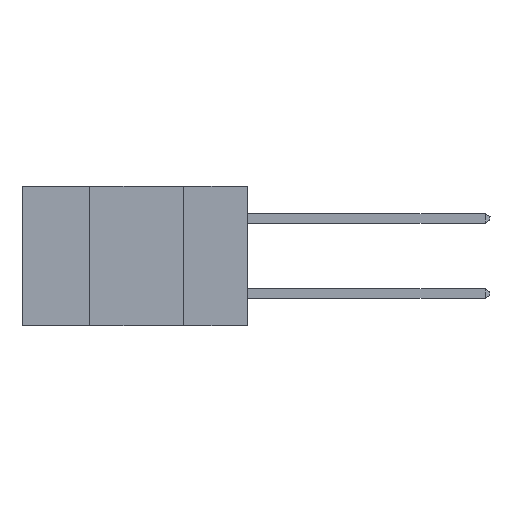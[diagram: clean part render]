
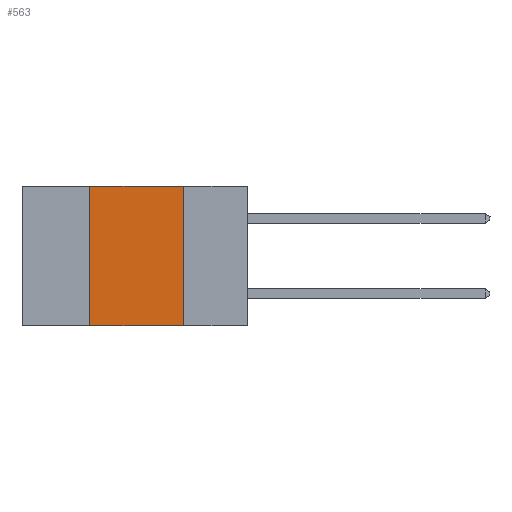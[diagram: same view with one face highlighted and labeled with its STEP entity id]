
A CAD part, left-side view. The second image highlights one B-rep face of the part: STEP entity #563.
In plain terms, the highlighted planar face has unit normal (-1, 0, 0).
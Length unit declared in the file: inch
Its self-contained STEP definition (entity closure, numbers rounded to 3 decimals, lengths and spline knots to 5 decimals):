
#563 = ADVANCED_FACE ( 'NONE', ( #631 ), #5371, .F. ) ;
#631 = FACE_OUTER_BOUND ( 'NONE', #15183, .T. ) ;
#861 = LINE ( 'NONE', #5600, #4841 ) ;
#929 = CARTESIAN_POINT ( 'NONE',  ( 0., 0.17, -0.37 ) ) ;
#1755 = ORIENTED_EDGE ( 'NONE', *, *, #13039, .F. ) ;
#1930 = LINE ( 'NONE', #14336, #5604 ) ;
#2170 = VERTEX_POINT ( 'NONE', #2237 ) ;
#2237 = CARTESIAN_POINT ( 'NONE',  ( 0., 0.42, -0.37 ) ) ;
#2641 = AXIS2_PLACEMENT_3D ( 'NONE', #10121, #14870, #3263 ) ;
#3263 = DIRECTION ( 'NONE',  ( 0., 0., -1. ) ) ;
#3550 = ORIENTED_EDGE ( 'NONE', *, *, #6660, .T. ) ;
#3672 = DIRECTION ( 'NONE',  ( 0., -1., 0. ) ) ;
#4181 = CARTESIAN_POINT ( 'NONE',  ( 0., 0.17, 0. ) ) ;
#4212 = LINE ( 'NONE', #929, #6232 ) ;
#4841 = VECTOR ( 'NONE', #6774, 39.37008 ) ;
#5371 = PLANE ( 'NONE',  #2641 ) ;
#5600 = CARTESIAN_POINT ( 'NONE',  ( 0., 0.42, -0.37 ) ) ;
#5604 = VECTOR ( 'NONE', #3672, 39.37008 ) ;
#6186 = CARTESIAN_POINT ( 'NONE',  ( 0., 0.6, 0. ) ) ;
#6232 = VECTOR ( 'NONE', #14010, 39.37008 ) ;
#6468 = ORIENTED_EDGE ( 'NONE', *, *, #8376, .F. ) ;
#6473 = VERTEX_POINT ( 'NONE', #4181 ) ;
#6573 = CARTESIAN_POINT ( 'NONE',  ( 0., 0.17, -0.37 ) ) ;
#6660 = EDGE_CURVE ( 'NONE', #2170, #8579, #1930, .T. ) ;
#6774 = DIRECTION ( 'NONE',  ( 0., 0., 1. ) ) ;
#8376 = EDGE_CURVE ( 'NONE', #15079, #6473, #13581, .T. ) ;
#8579 = VERTEX_POINT ( 'NONE', #6573 ) ;
#9232 = ORIENTED_EDGE ( 'NONE', *, *, #9540, .F. ) ;
#9540 = EDGE_CURVE ( 'NONE', #6473, #8579, #4212, .T. ) ;
#10121 = CARTESIAN_POINT ( 'NONE',  ( 0., 0.6, 0. ) ) ;
#11269 = VECTOR ( 'NONE', #14520, 39.37008 ) ;
#13039 = EDGE_CURVE ( 'NONE', #2170, #15079, #861, .T. ) ;
#13581 = LINE ( 'NONE', #6186, #11269 ) ;
#13732 = CARTESIAN_POINT ( 'NONE',  ( 0., 0.42, 0. ) ) ;
#14010 = DIRECTION ( 'NONE',  ( 0., 0., -1. ) ) ;
#14336 = CARTESIAN_POINT ( 'NONE',  ( 0., 0.6, -0.37 ) ) ;
#14520 = DIRECTION ( 'NONE',  ( 0., -1., 0. ) ) ;
#14870 = DIRECTION ( 'NONE',  ( 1., 0., 0. ) ) ;
#15079 = VERTEX_POINT ( 'NONE', #13732 ) ;
#15183 = EDGE_LOOP ( 'NONE', ( #9232, #6468, #1755, #3550 ) ) ;
